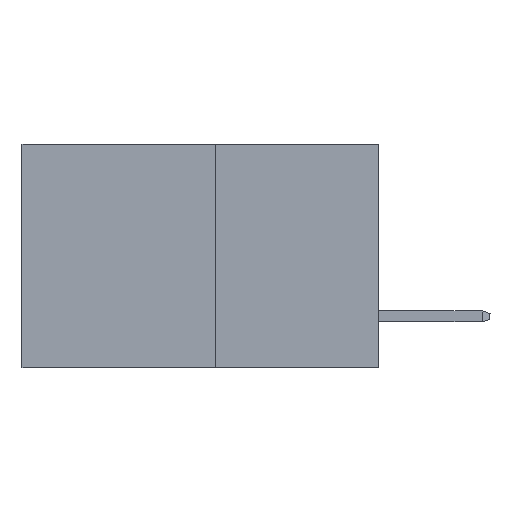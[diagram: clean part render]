
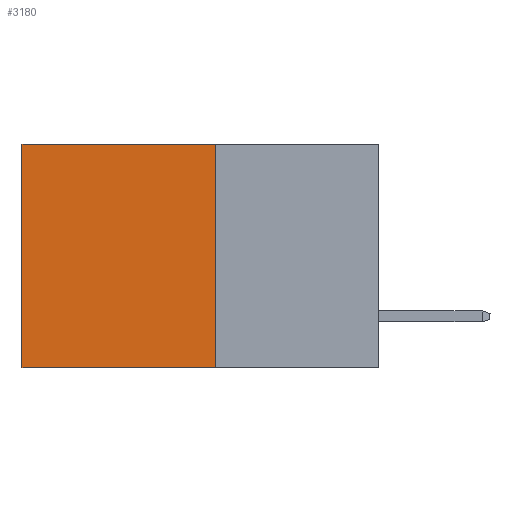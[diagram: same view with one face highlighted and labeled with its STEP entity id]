
A CAD part, left-side view. The second image highlights one B-rep face of the part: STEP entity #3180.
In plain terms, the highlighted planar face has unit normal (-1, 0, 0).
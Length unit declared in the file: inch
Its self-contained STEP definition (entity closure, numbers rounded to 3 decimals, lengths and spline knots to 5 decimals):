
#36 = ORIENTED_EDGE ( 'NONE', *, *, #10074, .T. ) ;
#259 = LINE ( 'NONE', #11545, #2230 ) ;
#280 = ORIENTED_EDGE ( 'NONE', *, *, #11540, .T. ) ;
#560 = EDGE_CURVE ( 'NONE', #2091, #5695, #7164, .T. ) ;
#696 = CARTESIAN_POINT ( 'NONE',  ( 0.277, 0.27, -0.37 ) ) ;
#744 = AXIS2_PLACEMENT_3D ( 'NONE', #8027, #6520, #7150 ) ;
#1869 = LINE ( 'NONE', #4668, #11053 ) ;
#2091 = VERTEX_POINT ( 'NONE', #696 ) ;
#2230 = VECTOR ( 'NONE', #11609, 39.37008 ) ;
#2287 = VECTOR ( 'NONE', #3378, 39.37008 ) ;
#3073 = CARTESIAN_POINT ( 'NONE',  ( 0.277, 0.27, 0. ) ) ;
#3180 = ADVANCED_FACE ( 'NONE', ( #10510 ), #4706, .F. ) ;
#3349 = CARTESIAN_POINT ( 'NONE',  ( 0.277, 0.27, -0.37 ) ) ;
#3378 = DIRECTION ( 'NONE',  ( 0., 1., 0. ) ) ;
#3511 = CARTESIAN_POINT ( 'NONE',  ( 0.277, 0.59, -0.37 ) ) ;
#3635 = EDGE_CURVE ( 'NONE', #5543, #2091, #259, .T. ) ;
#4668 = CARTESIAN_POINT ( 'NONE',  ( 0.277, 0.59, -0.37 ) ) ;
#4706 = PLANE ( 'NONE',  #744 ) ;
#5098 = EDGE_LOOP ( 'NONE', ( #36, #5896, #6238, #280 ) ) ;
#5543 = VERTEX_POINT ( 'NONE', #6322 ) ;
#5695 = VERTEX_POINT ( 'NONE', #3511 ) ;
#5896 = ORIENTED_EDGE ( 'NONE', *, *, #560, .F. ) ;
#6238 = ORIENTED_EDGE ( 'NONE', *, *, #3635, .F. ) ;
#6322 = CARTESIAN_POINT ( 'NONE',  ( 0.277, 0.27, 0. ) ) ;
#6520 = DIRECTION ( 'NONE',  ( 1., 0., 0. ) ) ;
#6703 = DIRECTION ( 'NONE',  ( 0., 1., 0. ) ) ;
#6907 = CARTESIAN_POINT ( 'NONE',  ( 0.277, 0.59, 0. ) ) ;
#7150 = DIRECTION ( 'NONE',  ( 0., 0., -1. ) ) ;
#7164 = LINE ( 'NONE', #3349, #2287 ) ;
#7827 = VECTOR ( 'NONE', #6703, 39.37008 ) ;
#8027 = CARTESIAN_POINT ( 'NONE',  ( 0.277, 0.27, -0.37 ) ) ;
#8200 = DIRECTION ( 'NONE',  ( 0., 0., -1. ) ) ;
#8476 = VERTEX_POINT ( 'NONE', #6907 ) ;
#9895 = LINE ( 'NONE', #3073, #7827 ) ;
#10074 = EDGE_CURVE ( 'NONE', #8476, #5695, #1869, .T. ) ;
#10510 = FACE_OUTER_BOUND ( 'NONE', #5098, .T. ) ;
#11053 = VECTOR ( 'NONE', #8200, 39.37008 ) ;
#11540 = EDGE_CURVE ( 'NONE', #5543, #8476, #9895, .T. ) ;
#11545 = CARTESIAN_POINT ( 'NONE',  ( 0.277, 0.27, -0.37 ) ) ;
#11609 = DIRECTION ( 'NONE',  ( 0., 0., -1. ) ) ;
